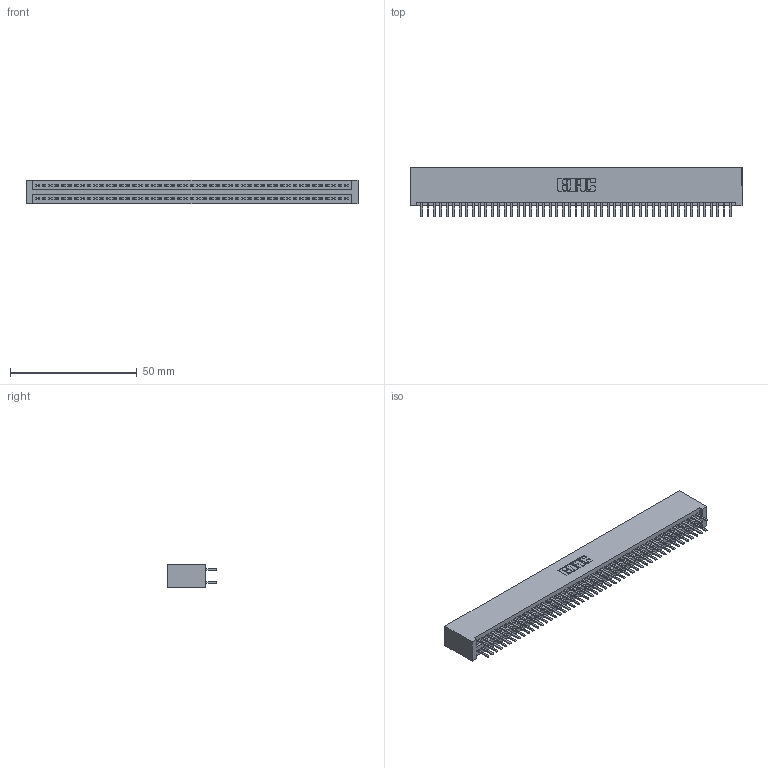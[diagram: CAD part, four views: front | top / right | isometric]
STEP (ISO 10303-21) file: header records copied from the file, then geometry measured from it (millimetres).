
FILE_DESCRIPTION (( 'STEP AP203' ), '1' );
FILE_NAME ('395-098-520-201.STEP', '2018-11-29T18:33:06', ( '' ), ( '' ), 'SwSTEP 2.0', 'SolidWorks 2016', '' );
FILE_SCHEMA (( 'CONFIG_CONTROL_DESIGN' ));
Length unit declared in the file: inch
Products named in the file (3): 345 Part_No Mounting Lugs; 395-098-520-201; 345-292-001_345-293-120
Assembly tree (99 placements, depth 2):
  395-098-520-201
    345 Part_No Mounting Lugs
    345-292-001_345-293-120  x98
Bounding box: 131.06 x 19.68 x 9.4 mm (x, y, z)
Volume: 13369.5 mm3; surface area: 20109.6 mm2
Topology: 99 solids, 99 shells, 5410 faces, 15703 edges, 10206 vertices
Faces by surface type: plane 3506, cylinder 1904
Entity records: 37341 total; most frequent: CARTESIAN_POINT 6264, ORIENTED_EDGE 6186, DIRECTION 5497, EDGE_CURVE 3093, LINE 2769, VECTOR 2769, VERTEX_POINT 2058, AXIS2_PLACEMENT_3D 1364
